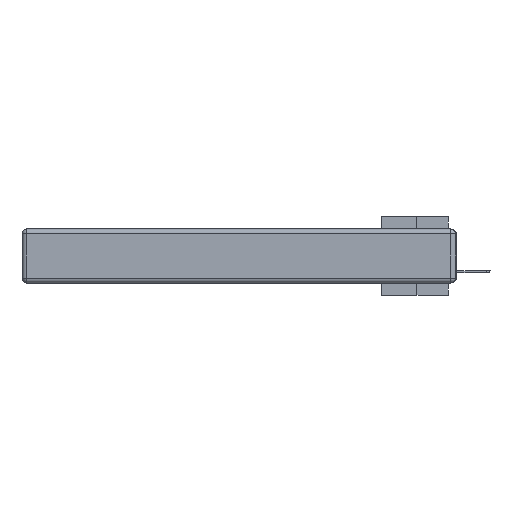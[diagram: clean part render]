
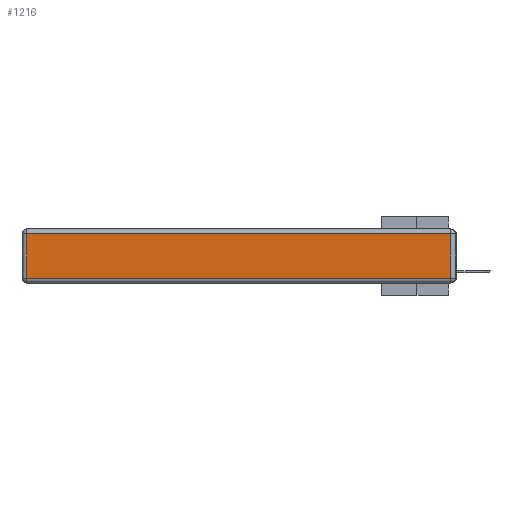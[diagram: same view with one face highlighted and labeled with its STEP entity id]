
A CAD part, left-side view. The second image highlights one B-rep face of the part: STEP entity #1216.
In plain terms, the highlighted planar face has unit normal (-1, 0, 0).
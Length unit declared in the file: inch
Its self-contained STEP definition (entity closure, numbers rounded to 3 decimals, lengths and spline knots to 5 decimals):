
#1216 = ADVANCED_FACE ( 'NONE', ( #32819 ), #11561, .T. ) ;
#4423 = ORIENTED_EDGE ( 'NONE', *, *, #24895, .T. ) ;
#4804 = VECTOR ( 'NONE', #6523, 39.37008 ) ;
#6523 = DIRECTION ( 'NONE',  ( 0., 0., -1. ) ) ;
#8004 = CARTESIAN_POINT ( 'NONE',  ( 0., 0.03, -0.343 ) ) ;
#8237 = CARTESIAN_POINT ( 'NONE',  ( 0., 0.03, -0.03 ) ) ;
#8490 = EDGE_CURVE ( 'NONE', #10657, #23586, #20742, .T. ) ;
#8771 = ORIENTED_EDGE ( 'NONE', *, *, #32749, .T. ) ;
#8807 = ORIENTED_EDGE ( 'NONE', *, *, #20011, .T. ) ;
#10657 = VERTEX_POINT ( 'NONE', #8237 ) ;
#10949 = AXIS2_PLACEMENT_3D ( 'NONE', #19879, #24291, #29579 ) ;
#11561 = PLANE ( 'NONE',  #10949 ) ;
#12139 = CARTESIAN_POINT ( 'NONE',  ( 0., 0.03, -0.313 ) ) ;
#12327 = ORIENTED_EDGE ( 'NONE', *, *, #8490, .T. ) ;
#12594 = DIRECTION ( 'NONE',  ( 0., 1., 0. ) ) ;
#12618 = DIRECTION ( 'NONE',  ( 0., -1., 0. ) ) ;
#14643 = CARTESIAN_POINT ( 'NONE',  ( 0., 2.72, -0.03 ) ) ;
#16119 = VECTOR ( 'NONE', #12618, 39.37008 ) ;
#16911 = CARTESIAN_POINT ( 'NONE',  ( 0., 2.72, -0.343 ) ) ;
#19879 = CARTESIAN_POINT ( 'NONE',  ( 0., 0., -0.343 ) ) ;
#20011 = EDGE_CURVE ( 'NONE', #30325, #10657, #20606, .T. ) ;
#20606 = LINE ( 'NONE', #8004, #22452 ) ;
#20742 = LINE ( 'NONE', #28567, #21143 ) ;
#21143 = VECTOR ( 'NONE', #12594, 39.37008 ) ;
#22452 = VECTOR ( 'NONE', #24262, 39.37008 ) ;
#23478 = CARTESIAN_POINT ( 'NONE',  ( 0., 0., -0.313 ) ) ;
#23586 = VERTEX_POINT ( 'NONE', #14643 ) ;
#24262 = DIRECTION ( 'NONE',  ( 0., 0., 1. ) ) ;
#24291 = DIRECTION ( 'NONE',  ( -1., 0., 0. ) ) ;
#24895 = EDGE_CURVE ( 'NONE', #26943, #30325, #33372, .T. ) ;
#26943 = VERTEX_POINT ( 'NONE', #32956 ) ;
#28567 = CARTESIAN_POINT ( 'NONE',  ( 0., 2.75, -0.03 ) ) ;
#29579 = DIRECTION ( 'NONE',  ( 0., 0., 1. ) ) ;
#29836 = LINE ( 'NONE', #16911, #4804 ) ;
#30325 = VERTEX_POINT ( 'NONE', #12139 ) ;
#32670 = EDGE_LOOP ( 'NONE', ( #4423, #8807, #12327, #8771 ) ) ;
#32749 = EDGE_CURVE ( 'NONE', #23586, #26943, #29836, .T. ) ;
#32819 = FACE_OUTER_BOUND ( 'NONE', #32670, .T. ) ;
#32956 = CARTESIAN_POINT ( 'NONE',  ( 0., 2.72, -0.313 ) ) ;
#33372 = LINE ( 'NONE', #23478, #16119 ) ;
